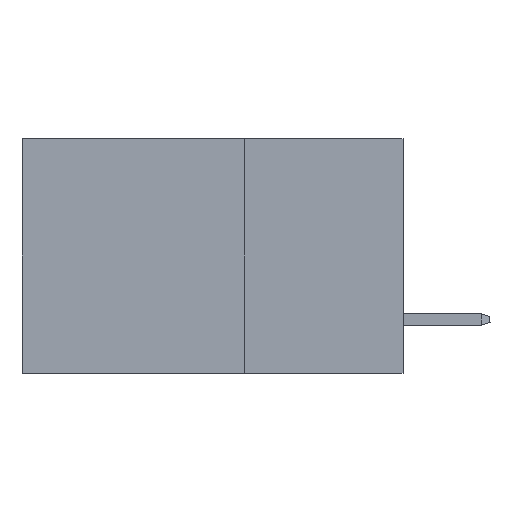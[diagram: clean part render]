
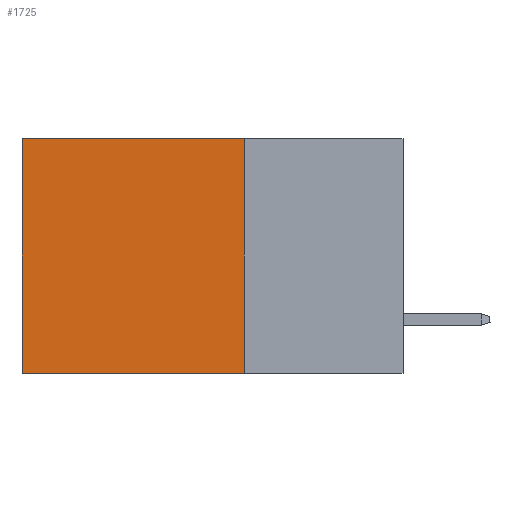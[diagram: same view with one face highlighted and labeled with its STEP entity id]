
A CAD part, left-side view. The second image highlights one B-rep face of the part: STEP entity #1725.
In plain terms, the highlighted planar face has unit normal (-1, 0, 0).
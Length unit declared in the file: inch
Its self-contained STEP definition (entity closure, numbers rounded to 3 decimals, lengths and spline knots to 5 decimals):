
#888 = EDGE_CURVE ( 'NONE', #41843, #12096, #11799, .T. ) ;
#944 = FACE_OUTER_BOUND ( 'NONE', #7790, .T. ) ;
#1725 = ADVANCED_FACE ( 'NONE', ( #944 ), #13869, .F. ) ;
#3836 = CARTESIAN_POINT ( 'NONE',  ( 0.2875, 0.6, -0.37 ) ) ;
#5414 = VECTOR ( 'NONE', #39273, 39.37008 ) ;
#7322 = VERTEX_POINT ( 'NONE', #21916 ) ;
#7790 = EDGE_LOOP ( 'NONE', ( #15457, #22601, #26145, #8807 ) ) ;
#8807 = ORIENTED_EDGE ( 'NONE', *, *, #32708, .T. ) ;
#8922 = DIRECTION ( 'NONE',  ( 0., 0., -1. ) ) ;
#9888 = VECTOR ( 'NONE', #8922, 39.37008 ) ;
#10642 = VECTOR ( 'NONE', #28820, 39.37008 ) ;
#10760 = EDGE_CURVE ( 'NONE', #18423, #7322, #36596, .T. ) ;
#11799 = LINE ( 'NONE', #35324, #9888 ) ;
#12096 = VERTEX_POINT ( 'NONE', #3836 ) ;
#13869 = PLANE ( 'NONE',  #20410 ) ;
#14713 = CARTESIAN_POINT ( 'NONE',  ( 0.2875, 0.25, 0. ) ) ;
#15457 = ORIENTED_EDGE ( 'NONE', *, *, #888, .T. ) ;
#16029 = LINE ( 'NONE', #33408, #19369 ) ;
#16778 = EDGE_CURVE ( 'NONE', #7322, #12096, #16029, .T. ) ;
#18423 = VERTEX_POINT ( 'NONE', #14713 ) ;
#19369 = VECTOR ( 'NONE', #29475, 39.37008 ) ;
#20410 = AXIS2_PLACEMENT_3D ( 'NONE', #27305, #20903, #23535 ) ;
#20903 = DIRECTION ( 'NONE',  ( 1., 0., 0. ) ) ;
#21916 = CARTESIAN_POINT ( 'NONE',  ( 0.2875, 0.25, -0.37 ) ) ;
#22601 = ORIENTED_EDGE ( 'NONE', *, *, #16778, .F. ) ;
#23535 = DIRECTION ( 'NONE',  ( 0., 0., -1. ) ) ;
#25929 = CARTESIAN_POINT ( 'NONE',  ( 0.2875, 0.25, 0. ) ) ;
#26145 = ORIENTED_EDGE ( 'NONE', *, *, #10760, .F. ) ;
#27305 = CARTESIAN_POINT ( 'NONE',  ( 0.2875, 0.25, 0. ) ) ;
#28820 = DIRECTION ( 'NONE',  ( 0., 1., 0. ) ) ;
#29475 = DIRECTION ( 'NONE',  ( 0., 1., 0. ) ) ;
#32708 = EDGE_CURVE ( 'NONE', #18423, #41843, #39360, .T. ) ;
#33408 = CARTESIAN_POINT ( 'NONE',  ( 0.2875, 0.25, -0.37 ) ) ;
#35324 = CARTESIAN_POINT ( 'NONE',  ( 0.2875, 0.6, 0. ) ) ;
#36596 = LINE ( 'NONE', #42778, #5414 ) ;
#39273 = DIRECTION ( 'NONE',  ( 0., 0., -1. ) ) ;
#39360 = LINE ( 'NONE', #25929, #10642 ) ;
#41843 = VERTEX_POINT ( 'NONE', #42016 ) ;
#42016 = CARTESIAN_POINT ( 'NONE',  ( 0.2875, 0.6, 0. ) ) ;
#42778 = CARTESIAN_POINT ( 'NONE',  ( 0.2875, 0.25, 0. ) ) ;
